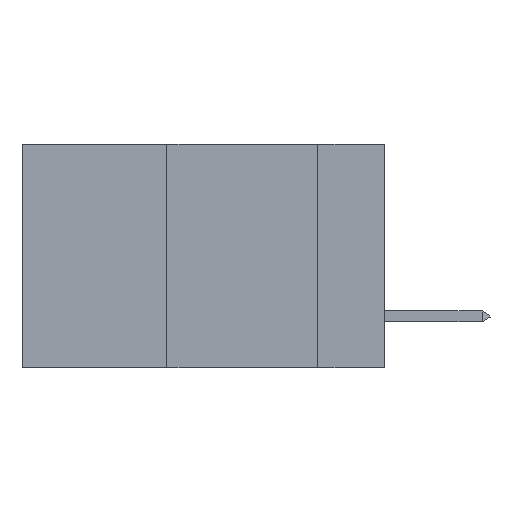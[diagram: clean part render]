
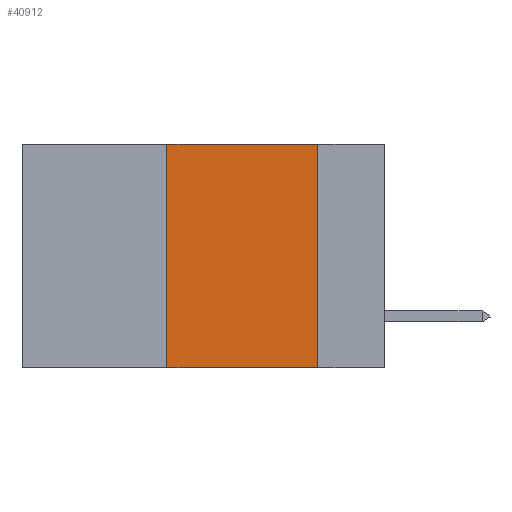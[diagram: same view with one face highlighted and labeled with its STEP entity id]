
A CAD part, left-side view. The second image highlights one B-rep face of the part: STEP entity #40912.
In plain terms, the highlighted planar face has unit normal (-1, 0, 0).
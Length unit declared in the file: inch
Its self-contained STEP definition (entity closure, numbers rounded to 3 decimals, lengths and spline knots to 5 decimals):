
#947 = CARTESIAN_POINT ( 'NONE',  ( 0., 0.11, -0.37 ) ) ;
#1595 = DIRECTION ( 'NONE',  ( 0., -1., 0. ) ) ;
#2027 = CARTESIAN_POINT ( 'NONE',  ( 0., 0.36, -0.37 ) ) ;
#2395 = EDGE_CURVE ( 'NONE', #23239, #5557, #29601, .T. ) ;
#2502 = VERTEX_POINT ( 'NONE', #2027 ) ;
#2577 = DIRECTION ( 'NONE',  ( 0., -1., 0. ) ) ;
#2611 = VECTOR ( 'NONE', #1595, 39.37008 ) ;
#2618 = DIRECTION ( 'NONE',  ( 0., 0., 1. ) ) ;
#4010 = CARTESIAN_POINT ( 'NONE',  ( 0., 0.36, 0. ) ) ;
#4427 = LINE ( 'NONE', #18962, #23656 ) ;
#4933 = CARTESIAN_POINT ( 'NONE',  ( 0., 0.6, 0. ) ) ;
#5094 = EDGE_LOOP ( 'NONE', ( #41894, #34159, #6854, #30516 ) ) ;
#5557 = VERTEX_POINT ( 'NONE', #38668 ) ;
#5558 = DIRECTION ( 'NONE',  ( 0., 0., -1. ) ) ;
#6854 = ORIENTED_EDGE ( 'NONE', *, *, #35243, .F. ) ;
#7219 = AXIS2_PLACEMENT_3D ( 'NONE', #24283, #37592, #5558 ) ;
#8026 = FACE_OUTER_BOUND ( 'NONE', #5094, .T. ) ;
#9040 = EDGE_CURVE ( 'NONE', #5557, #9764, #4427, .T. ) ;
#9764 = VERTEX_POINT ( 'NONE', #947 ) ;
#12441 = CARTESIAN_POINT ( 'NONE',  ( 0., 0.36, 0. ) ) ;
#18962 = CARTESIAN_POINT ( 'NONE',  ( 0., 0.11, 0. ) ) ;
#19034 = CARTESIAN_POINT ( 'NONE',  ( 0., 0.6, -0.37 ) ) ;
#21800 = DIRECTION ( 'NONE',  ( 0., 0., -1. ) ) ;
#23239 = VERTEX_POINT ( 'NONE', #4010 ) ;
#23656 = VECTOR ( 'NONE', #21800, 39.37008 ) ;
#24283 = CARTESIAN_POINT ( 'NONE',  ( 0., 0.6, 0. ) ) ;
#24770 = PLANE ( 'NONE',  #7219 ) ;
#27901 = LINE ( 'NONE', #19034, #31541 ) ;
#28958 = EDGE_CURVE ( 'NONE', #2502, #9764, #27901, .T. ) ;
#29601 = LINE ( 'NONE', #4933, #2611 ) ;
#30516 = ORIENTED_EDGE ( 'NONE', *, *, #28958, .T. ) ;
#31541 = VECTOR ( 'NONE', #2577, 39.37008 ) ;
#34159 = ORIENTED_EDGE ( 'NONE', *, *, #2395, .F. ) ;
#35243 = EDGE_CURVE ( 'NONE', #2502, #23239, #36149, .T. ) ;
#35624 = VECTOR ( 'NONE', #2618, 39.37008 ) ;
#36149 = LINE ( 'NONE', #12441, #35624 ) ;
#37592 = DIRECTION ( 'NONE',  ( 1., 0., 0. ) ) ;
#38668 = CARTESIAN_POINT ( 'NONE',  ( 0., 0.11, 0. ) ) ;
#40912 = ADVANCED_FACE ( 'NONE', ( #8026 ), #24770, .F. ) ;
#41894 = ORIENTED_EDGE ( 'NONE', *, *, #9040, .F. ) ;
